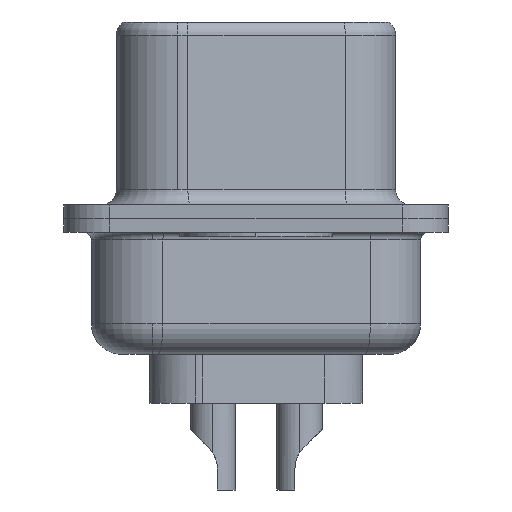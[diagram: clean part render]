
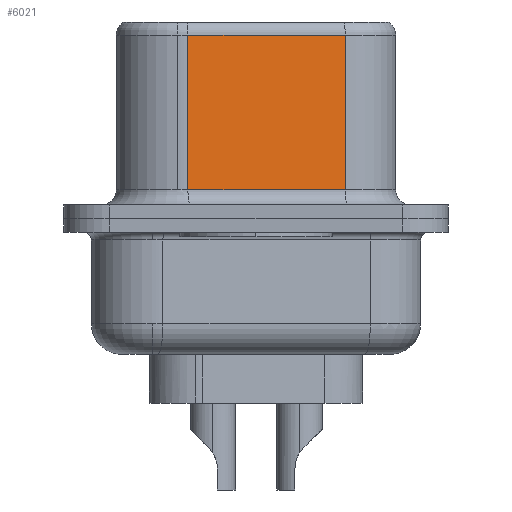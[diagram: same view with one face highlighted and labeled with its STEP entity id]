
A CAD part, left-side view. The second image highlights one B-rep face of the part: STEP entity #6021.
In plain terms, the highlighted planar face has unit normal (-0.985, -0.174, 0).
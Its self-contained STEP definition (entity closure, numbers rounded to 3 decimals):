
#252 = VERTEX_POINT ( 'NONE', #7681 ) ;
#565 = DIRECTION ( 'NONE',  ( 0., 0., -1. ) ) ;
#651 = DIRECTION ( 'NONE',  ( 0., 0., -1. ) ) ;
#704 = CARTESIAN_POINT ( 'NONE',  ( 3.665, 2.233, 0.95 ) ) ;
#1180 = DIRECTION ( 'NONE',  ( 0.985, 0.174, 0. ) ) ;
#1309 = AXIS2_PLACEMENT_3D ( 'NONE', #13284, #1180, #7765 ) ;
#1704 = LINE ( 'NONE', #10543, #1749 ) ;
#1749 = VECTOR ( 'NONE', #2854, 1000. ) ;
#2659 = LINE ( 'NONE', #3807, #9890 ) ;
#2854 = DIRECTION ( 'NONE',  ( 0.174, -0.985, 0. ) ) ;
#2911 = ORIENTED_EDGE ( 'NONE', *, *, #9014, .T. ) ;
#2951 = EDGE_CURVE ( 'NONE', #252, #8205, #6751, .T. ) ;
#3300 = VECTOR ( 'NONE', #6978, 1000. ) ;
#3344 = VECTOR ( 'NONE', #651, 1000. ) ;
#3807 = CARTESIAN_POINT ( 'NONE',  ( 4.575, -2.927, 6.52 ) ) ;
#4886 = VERTEX_POINT ( 'NONE', #12704 ) ;
#5732 = CARTESIAN_POINT ( 'NONE',  ( 4.575, -2.927, 6.02 ) ) ;
#6021 = ADVANCED_FACE ( 'NONE', ( #10889 ), #8704, .F. ) ;
#6077 = LINE ( 'NONE', #10576, #3344 ) ;
#6751 = LINE ( 'NONE', #5732, #3300 ) ;
#6978 = DIRECTION ( 'NONE',  ( -0.174, 0.985, 0. ) ) ;
#7681 = CARTESIAN_POINT ( 'NONE',  ( 4.575, -2.927, 6.02 ) ) ;
#7765 = DIRECTION ( 'NONE',  ( -0.174, 0.985, 0. ) ) ;
#8205 = VERTEX_POINT ( 'NONE', #11581 ) ;
#8704 = PLANE ( 'NONE',  #1309 ) ;
#9014 = EDGE_CURVE ( 'NONE', #8205, #11495, #6077, .T. ) ;
#9857 = EDGE_CURVE ( 'NONE', #11495, #4886, #1704, .T. ) ;
#9890 = VECTOR ( 'NONE', #565, 1000. ) ;
#10543 = CARTESIAN_POINT ( 'NONE',  ( 4.575, -2.927, 0.95 ) ) ;
#10576 = CARTESIAN_POINT ( 'NONE',  ( 3.665, 2.233, 6.52 ) ) ;
#10763 = ORIENTED_EDGE ( 'NONE', *, *, #9857, .T. ) ;
#10889 = FACE_OUTER_BOUND ( 'NONE', #13512, .T. ) ;
#11495 = VERTEX_POINT ( 'NONE', #704 ) ;
#11581 = CARTESIAN_POINT ( 'NONE',  ( 3.665, 2.233, 6.02 ) ) ;
#12420 = ORIENTED_EDGE ( 'NONE', *, *, #2951, .T. ) ;
#12577 = EDGE_CURVE ( 'NONE', #252, #4886, #2659, .T. ) ;
#12704 = CARTESIAN_POINT ( 'NONE',  ( 4.575, -2.927, 0.95 ) ) ;
#12711 = ORIENTED_EDGE ( 'NONE', *, *, #12577, .F. ) ;
#13284 = CARTESIAN_POINT ( 'NONE',  ( 4.575, -2.927, 6.52 ) ) ;
#13512 = EDGE_LOOP ( 'NONE', ( #12711, #12420, #2911, #10763 ) ) ;
